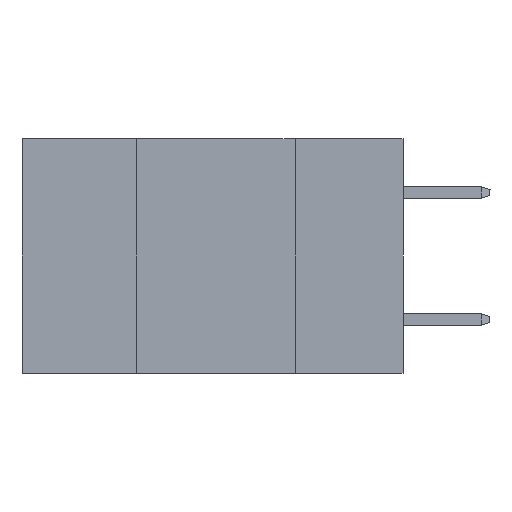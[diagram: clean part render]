
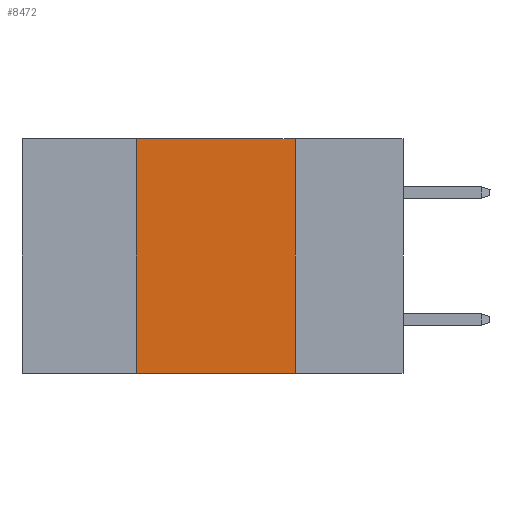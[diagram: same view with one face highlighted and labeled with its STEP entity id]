
A CAD part, left-side view. The second image highlights one B-rep face of the part: STEP entity #8472.
In plain terms, the highlighted planar face has unit normal (-1, 0, 0).
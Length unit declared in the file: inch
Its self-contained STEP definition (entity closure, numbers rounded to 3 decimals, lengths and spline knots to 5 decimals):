
#1614 = VECTOR ( 'NONE', #11880, 39.37008 ) ;
#2063 = EDGE_CURVE ( 'NONE', #23327, #13482, #22408, .T. ) ;
#2400 = ORIENTED_EDGE ( 'NONE', *, *, #2063, .F. ) ;
#3463 = CARTESIAN_POINT ( 'NONE',  ( 0., 0.42, 0. ) ) ;
#5669 = VERTEX_POINT ( 'NONE', #15822 ) ;
#5769 = VECTOR ( 'NONE', #13214, 39.37008 ) ;
#5774 = CARTESIAN_POINT ( 'NONE',  ( 0., 0.6, 0. ) ) ;
#6915 = EDGE_LOOP ( 'NONE', ( #20474, #13292, #2400, #24629 ) ) ;
#8472 = ADVANCED_FACE ( 'NONE', ( #10013 ), #14319, .F. ) ;
#9208 = VERTEX_POINT ( 'NONE', #18127 ) ;
#10013 = FACE_OUTER_BOUND ( 'NONE', #6915, .T. ) ;
#10635 = CARTESIAN_POINT ( 'NONE',  ( 0., 0.17, 0. ) ) ;
#11880 = DIRECTION ( 'NONE',  ( 0., 0., 1. ) ) ;
#12044 = DIRECTION ( 'NONE',  ( 0., -1., 0. ) ) ;
#13214 = DIRECTION ( 'NONE',  ( 0., -1., 0. ) ) ;
#13292 = ORIENTED_EDGE ( 'NONE', *, *, #21645, .F. ) ;
#13482 = VERTEX_POINT ( 'NONE', #21646 ) ;
#14031 = VECTOR ( 'NONE', #12044, 39.37008 ) ;
#14047 = DIRECTION ( 'NONE',  ( 1., 0., 0. ) ) ;
#14131 = LINE ( 'NONE', #16343, #14031 ) ;
#14319 = PLANE ( 'NONE',  #26518 ) ;
#14545 = EDGE_CURVE ( 'NONE', #23327, #5669, #14131, .T. ) ;
#15822 = CARTESIAN_POINT ( 'NONE',  ( 0., 0.17, -0.37 ) ) ;
#16343 = CARTESIAN_POINT ( 'NONE',  ( 0., 0.6, -0.37 ) ) ;
#16806 = VECTOR ( 'NONE', #18939, 39.37008 ) ;
#17381 = CARTESIAN_POINT ( 'NONE',  ( 0., 0.42, -0.37 ) ) ;
#18127 = CARTESIAN_POINT ( 'NONE',  ( 0., 0.17, 0. ) ) ;
#18939 = DIRECTION ( 'NONE',  ( 0., 0., -1. ) ) ;
#19574 = LINE ( 'NONE', #26233, #5769 ) ;
#20474 = ORIENTED_EDGE ( 'NONE', *, *, #27329, .F. ) ;
#21010 = LINE ( 'NONE', #10635, #16806 ) ;
#21645 = EDGE_CURVE ( 'NONE', #13482, #9208, #19574, .T. ) ;
#21646 = CARTESIAN_POINT ( 'NONE',  ( 0., 0.42, 0. ) ) ;
#22408 = LINE ( 'NONE', #3463, #1614 ) ;
#22492 = DIRECTION ( 'NONE',  ( 0., 0., -1. ) ) ;
#23327 = VERTEX_POINT ( 'NONE', #17381 ) ;
#24629 = ORIENTED_EDGE ( 'NONE', *, *, #14545, .T. ) ;
#26233 = CARTESIAN_POINT ( 'NONE',  ( 0., 0.6, 0. ) ) ;
#26518 = AXIS2_PLACEMENT_3D ( 'NONE', #5774, #14047, #22492 ) ;
#27329 = EDGE_CURVE ( 'NONE', #9208, #5669, #21010, .T. ) ;
